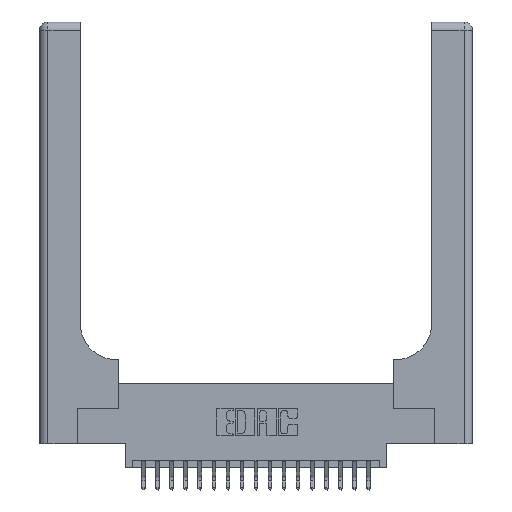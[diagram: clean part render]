
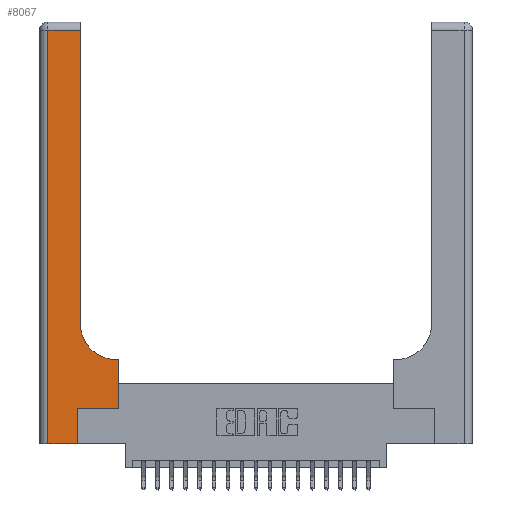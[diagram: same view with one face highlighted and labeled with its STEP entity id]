
A CAD part, top view. The second image highlights one B-rep face of the part: STEP entity #8067.
In plain terms, the highlighted planar face has unit normal (0, 0, 1).
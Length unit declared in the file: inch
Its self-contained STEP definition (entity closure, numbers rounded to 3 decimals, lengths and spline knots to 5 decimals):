
#1029 = CARTESIAN_POINT ( 'NONE',  ( 0.2915, 2.94, 0.37 ) ) ;
#1331 = LINE ( 'NONE', #13689, #11121 ) ;
#1447 = ORIENTED_EDGE ( 'NONE', *, *, #20484, .T. ) ;
#1601 = DIRECTION ( 'NONE',  ( 0., -1., 0. ) ) ;
#1766 = AXIS2_PLACEMENT_3D ( 'NONE', #5876, #17830, #7657 ) ;
#1854 = VERTEX_POINT ( 'NONE', #12601 ) ;
#2795 = DIRECTION ( 'NONE',  ( 0., 1., 0. ) ) ;
#3255 = LINE ( 'NONE', #4225, #20980 ) ;
#3479 = VECTOR ( 'NONE', #17659, 39.37008 ) ;
#4225 = CARTESIAN_POINT ( 'NONE',  ( 0., 0., 0.37 ) ) ;
#4302 = DIRECTION ( 'NONE',  ( 1., 0., 0. ) ) ;
#4507 = DIRECTION ( 'NONE',  ( 0., 0., -1. ) ) ;
#5293 = EDGE_CURVE ( 'NONE', #8076, #15722, #21338, .T. ) ;
#5369 = ORIENTED_EDGE ( 'NONE', *, *, #19841, .T. ) ;
#5425 = CARTESIAN_POINT ( 'NONE',  ( 0.269, 0.25, 0.37 ) ) ;
#5876 = CARTESIAN_POINT ( 'NONE',  ( 0.5415, 0.85, 0.37 ) ) ;
#6143 = AXIS2_PLACEMENT_3D ( 'NONE', #11333, #4507, #16511 ) ;
#6478 = ORIENTED_EDGE ( 'NONE', *, *, #6786, .T. ) ;
#6771 = EDGE_CURVE ( 'NONE', #18470, #18379, #8224, .T. ) ;
#6786 = EDGE_CURVE ( 'NONE', #18379, #21460, #12205, .T. ) ;
#7551 = VECTOR ( 'NONE', #21143, 39.37008 ) ;
#7657 = DIRECTION ( 'NONE',  ( 1., 0., 0. ) ) ;
#8067 = ADVANCED_FACE ( 'NONE', ( #11664 ), #14843, .F. ) ;
#8076 = VERTEX_POINT ( 'NONE', #19949 ) ;
#8224 = LINE ( 'NONE', #14886, #9296 ) ;
#8288 = VECTOR ( 'NONE', #13068, 39.37008 ) ;
#8570 = ORIENTED_EDGE ( 'NONE', *, *, #6771, .T. ) ;
#9296 = VECTOR ( 'NONE', #2795, 39.37008 ) ;
#9690 = ORIENTED_EDGE ( 'NONE', *, *, #5293, .T. ) ;
#10955 = EDGE_LOOP ( 'NONE', ( #16207, #12487, #12425, #12050, #9690, #1447, #8570, #6478, #5369 ) ) ;
#11121 = VECTOR ( 'NONE', #1601, 39.37008 ) ;
#11333 = CARTESIAN_POINT ( 'NONE',  ( 0., 3., 0.37 ) ) ;
#11379 = CARTESIAN_POINT ( 'NONE',  ( 0.269, 0., 0.37 ) ) ;
#11394 = CARTESIAN_POINT ( 'NONE',  ( 0.5585, 0.6, 0.37 ) ) ;
#11664 = FACE_OUTER_BOUND ( 'NONE', #10955, .T. ) ;
#12050 = ORIENTED_EDGE ( 'NONE', *, *, #19338, .T. ) ;
#12074 = VECTOR ( 'NONE', #15681, 39.37008 ) ;
#12096 = LINE ( 'NONE', #19421, #7551 ) ;
#12205 = LINE ( 'NONE', #19933, #20733 ) ;
#12425 = ORIENTED_EDGE ( 'NONE', *, *, #19672, .T. ) ;
#12487 = ORIENTED_EDGE ( 'NONE', *, *, #21923, .T. ) ;
#12601 = CARTESIAN_POINT ( 'NONE',  ( 0.06, 2.94, 0.37 ) ) ;
#13068 = DIRECTION ( 'NONE',  ( 0., 1., 0. ) ) ;
#13383 = CARTESIAN_POINT ( 'NONE',  ( 0.5585, 0.25, 0.37 ) ) ;
#13689 = CARTESIAN_POINT ( 'NONE',  ( 0.06, 3., 0.37 ) ) ;
#13728 = LINE ( 'NONE', #19323, #3479 ) ;
#13977 = CARTESIAN_POINT ( 'NONE',  ( 0., 2.94, 0.37 ) ) ;
#14843 = PLANE ( 'NONE',  #6143 ) ;
#14886 = CARTESIAN_POINT ( 'NONE',  ( 0.5585, 0.25, 0.37 ) ) ;
#15277 = VERTEX_POINT ( 'NONE', #19593 ) ;
#15405 = VERTEX_POINT ( 'NONE', #1029 ) ;
#15681 = DIRECTION ( 'NONE',  ( -1., 0., 0. ) ) ;
#15722 = VERTEX_POINT ( 'NONE', #5425 ) ;
#16207 = ORIENTED_EDGE ( 'NONE', *, *, #21459, .T. ) ;
#16511 = DIRECTION ( 'NONE',  ( -1., 0., 0. ) ) ;
#17105 = LINE ( 'NONE', #13977, #12074 ) ;
#17659 = DIRECTION ( 'NONE',  ( 1., 0., 0. ) ) ;
#17680 = CARTESIAN_POINT ( 'NONE',  ( 0.5415, 0.6, 0.37 ) ) ;
#17830 = DIRECTION ( 'NONE',  ( 0., 0., -1. ) ) ;
#18379 = VERTEX_POINT ( 'NONE', #11394 ) ;
#18470 = VERTEX_POINT ( 'NONE', #13383 ) ;
#18675 = CARTESIAN_POINT ( 'NONE',  ( 0.2915, 0.85, 0.37 ) ) ;
#19323 = CARTESIAN_POINT ( 'NONE',  ( 0.269, 0.25, 0.37 ) ) ;
#19338 = EDGE_CURVE ( 'NONE', #15277, #8076, #3255, .T. ) ;
#19421 = CARTESIAN_POINT ( 'NONE',  ( 0.2915, 3., 0.37 ) ) ;
#19593 = CARTESIAN_POINT ( 'NONE',  ( 0.06, 0., 0.37 ) ) ;
#19672 = EDGE_CURVE ( 'NONE', #1854, #15277, #1331, .T. ) ;
#19841 = EDGE_CURVE ( 'NONE', #21460, #21174, #20959, .T. ) ;
#19933 = CARTESIAN_POINT ( 'NONE',  ( 0.2915, 0.6, 0.37 ) ) ;
#19949 = CARTESIAN_POINT ( 'NONE',  ( 0.269, 0., 0.37 ) ) ;
#19997 = DIRECTION ( 'NONE',  ( -1., 0., 0. ) ) ;
#20484 = EDGE_CURVE ( 'NONE', #15722, #18470, #13728, .T. ) ;
#20733 = VECTOR ( 'NONE', #19997, 39.37008 ) ;
#20959 = CIRCLE ( 'NONE', #1766, 0.25 ) ;
#20980 = VECTOR ( 'NONE', #4302, 39.37008 ) ;
#21143 = DIRECTION ( 'NONE',  ( 0., 1., 0. ) ) ;
#21174 = VERTEX_POINT ( 'NONE', #18675 ) ;
#21338 = LINE ( 'NONE', #11379, #8288 ) ;
#21459 = EDGE_CURVE ( 'NONE', #21174, #15405, #12096, .T. ) ;
#21460 = VERTEX_POINT ( 'NONE', #17680 ) ;
#21923 = EDGE_CURVE ( 'NONE', #15405, #1854, #17105, .T. ) ;
